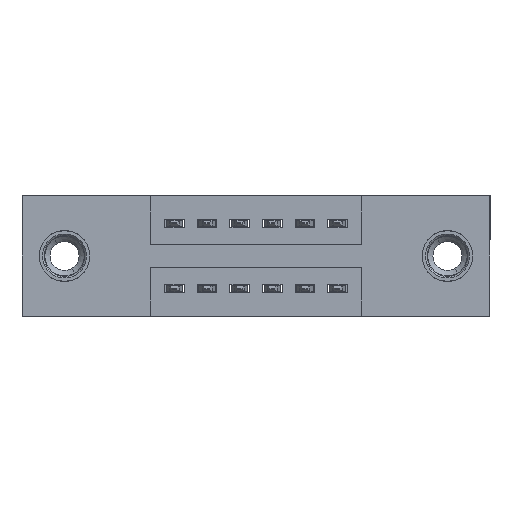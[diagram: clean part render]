
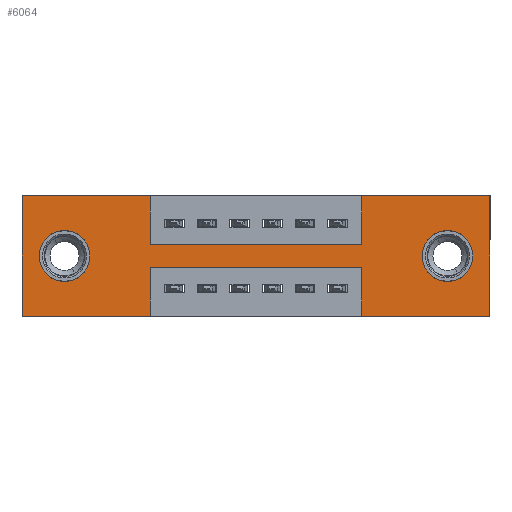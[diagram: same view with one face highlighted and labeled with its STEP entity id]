
A CAD part, front view. The second image highlights one B-rep face of the part: STEP entity #6064.
In plain terms, the highlighted planar face has unit normal (0, -1, 0).
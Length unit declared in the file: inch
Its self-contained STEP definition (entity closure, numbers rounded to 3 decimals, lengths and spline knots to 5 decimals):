
#124 = DIRECTION ( 'NONE',  ( 1., 0., 0. ) ) ;
#131 = LINE ( 'NONE', #4079, #9655 ) ;
#132 = EDGE_CURVE ( 'NONE', #5124, #314, #8219, .T. ) ;
#210 = ORIENTED_EDGE ( 'NONE', *, *, #3829, .T. ) ;
#260 = VECTOR ( 'NONE', #7945, 39.37008 ) ;
#314 = VERTEX_POINT ( 'NONE', #3733 ) ;
#321 = VERTEX_POINT ( 'NONE', #10904 ) ;
#384 = VERTEX_POINT ( 'NONE', #8227 ) ;
#517 = CARTESIAN_POINT ( 'NONE',  ( 1.0425, 0., -0.37 ) ) ;
#525 = EDGE_LOOP ( 'NONE', ( #11361, #210 ) ) ;
#572 = ORIENTED_EDGE ( 'NONE', *, *, #3975, .F. ) ;
#603 = CARTESIAN_POINT ( 'NONE',  ( 1.305, 0., -0.263 ) ) ;
#633 = AXIS2_PLACEMENT_3D ( 'NONE', #4261, #10539, #5156 ) ;
#740 = CIRCLE ( 'NONE', #633, 0.078 ) ;
#840 = CARTESIAN_POINT ( 'NONE',  ( 1.435, 0., 0. ) ) ;
#897 = DIRECTION ( 'NONE',  ( 0., -1., 0. ) ) ;
#974 = CARTESIAN_POINT ( 'NONE',  ( 0., 0., -0.37 ) ) ;
#1023 = ORIENTED_EDGE ( 'NONE', *, *, #4430, .T. ) ;
#1068 = DIRECTION ( 'NONE',  ( 0., 0., -1. ) ) ;
#1197 = LINE ( 'NONE', #10492, #3129 ) ;
#1275 = DIRECTION ( 'NONE',  ( 0., 1., 0. ) ) ;
#1791 = CARTESIAN_POINT ( 'NONE',  ( 0.3925, 0., 0. ) ) ;
#1823 = ORIENTED_EDGE ( 'NONE', *, *, #5217, .F. ) ;
#1884 = VERTEX_POINT ( 'NONE', #4316 ) ;
#1911 = VECTOR ( 'NONE', #6548, 39.37008 ) ;
#2116 = EDGE_CURVE ( 'NONE', #11554, #9631, #9535, .T. ) ;
#2135 = EDGE_CURVE ( 'NONE', #5106, #6953, #5011, .T. ) ;
#2216 = LINE ( 'NONE', #974, #1911 ) ;
#2228 = DIRECTION ( 'NONE',  ( 0., 1., 0. ) ) ;
#2556 = LINE ( 'NONE', #517, #260 ) ;
#2621 = VECTOR ( 'NONE', #3770, 39.37008 ) ;
#2711 = VECTOR ( 'NONE', #6985, 39.37008 ) ;
#2813 = ORIENTED_EDGE ( 'NONE', *, *, #6141, .F. ) ;
#2816 = EDGE_CURVE ( 'NONE', #314, #321, #131, .T. ) ;
#2923 = DIRECTION ( 'NONE',  ( 0., 0., -1. ) ) ;
#3078 = VECTOR ( 'NONE', #5081, 39.37008 ) ;
#3116 = CIRCLE ( 'NONE', #3929, 0.078 ) ;
#3129 = VECTOR ( 'NONE', #4170, 39.37008 ) ;
#3727 = CARTESIAN_POINT ( 'NONE',  ( 0., 0., -0.37 ) ) ;
#3733 = CARTESIAN_POINT ( 'NONE',  ( 0.3925, 0., -0.22 ) ) ;
#3770 = DIRECTION ( 'NONE',  ( 1., 0., 0. ) ) ;
#3829 = EDGE_CURVE ( 'NONE', #9293, #8934, #11154, .T. ) ;
#3920 = EDGE_CURVE ( 'NONE', #8699, #5106, #1197, .T. ) ;
#3929 = AXIS2_PLACEMENT_3D ( 'NONE', #6838, #1275, #7749 ) ;
#3975 = EDGE_CURVE ( 'NONE', #9783, #5124, #2556, .T. ) ;
#3978 = CARTESIAN_POINT ( 'NONE',  ( 0., 0., 0. ) ) ;
#4079 = CARTESIAN_POINT ( 'NONE',  ( 0.3925, 0., -0.37 ) ) ;
#4170 = DIRECTION ( 'NONE',  ( 1., 0., 0. ) ) ;
#4261 = CARTESIAN_POINT ( 'NONE',  ( 0.13, 0., -0.185 ) ) ;
#4316 = CARTESIAN_POINT ( 'NONE',  ( 1.0425, 0., -0.15 ) ) ;
#4330 = DIRECTION ( 'NONE',  ( -1., 0., 0. ) ) ;
#4430 = EDGE_CURVE ( 'NONE', #10887, #6436, #3116, .T. ) ;
#4585 = CARTESIAN_POINT ( 'NONE',  ( 1.0425, 0., -0.37 ) ) ;
#4748 = VECTOR ( 'NONE', #1068, 39.37008 ) ;
#4793 = ORIENTED_EDGE ( 'NONE', *, *, #2135, .F. ) ;
#4940 = FACE_BOUND ( 'NONE', #10703, .T. ) ;
#5011 = LINE ( 'NONE', #840, #4748 ) ;
#5038 = LINE ( 'NONE', #6460, #2621 ) ;
#5081 = DIRECTION ( 'NONE',  ( -1., 0., 0. ) ) ;
#5106 = VERTEX_POINT ( 'NONE', #10468 ) ;
#5108 = VECTOR ( 'NONE', #9379, 39.37008 ) ;
#5124 = VERTEX_POINT ( 'NONE', #10499 ) ;
#5156 = DIRECTION ( 'NONE',  ( 0., 0., 1. ) ) ;
#5217 = EDGE_CURVE ( 'NONE', #6953, #9783, #8957, .T. ) ;
#5424 = ORIENTED_EDGE ( 'NONE', *, *, #10143, .T. ) ;
#5445 = CARTESIAN_POINT ( 'NONE',  ( 1.305, 0., -0.185 ) ) ;
#5556 = EDGE_CURVE ( 'NONE', #384, #11554, #10025, .T. ) ;
#5749 = CARTESIAN_POINT ( 'NONE',  ( 0., 0., 0. ) ) ;
#6064 = ADVANCED_FACE ( 'NONE', ( #11798, #4940, #7673 ), #6459, .T. ) ;
#6141 = EDGE_CURVE ( 'NONE', #321, #10696, #2216, .T. ) ;
#6148 = CARTESIAN_POINT ( 'NONE',  ( 0., 0., -0.37 ) ) ;
#6224 = ORIENTED_EDGE ( 'NONE', *, *, #132, .F. ) ;
#6347 = DIRECTION ( 'NONE',  ( 0., 0., -1. ) ) ;
#6409 = ORIENTED_EDGE ( 'NONE', *, *, #3920, .F. ) ;
#6436 = VERTEX_POINT ( 'NONE', #7156 ) ;
#6459 = PLANE ( 'NONE',  #8289 ) ;
#6460 = CARTESIAN_POINT ( 'NONE',  ( 0.3925, 0., -0.15 ) ) ;
#6548 = DIRECTION ( 'NONE',  ( -1., 0., 0. ) ) ;
#6838 = CARTESIAN_POINT ( 'NONE',  ( 0.13, 0., -0.185 ) ) ;
#6940 = CARTESIAN_POINT ( 'NONE',  ( 1.0425, 0., 0. ) ) ;
#6953 = VERTEX_POINT ( 'NONE', #7176 ) ;
#6985 = DIRECTION ( 'NONE',  ( 0., 0., 1. ) ) ;
#7033 = EDGE_CURVE ( 'NONE', #8934, #9293, #7363, .T. ) ;
#7156 = CARTESIAN_POINT ( 'NONE',  ( 0.13, 0., -0.107 ) ) ;
#7157 = EDGE_LOOP ( 'NONE', ( #7839, #6224, #572, #1823, #4793, #6409, #11469, #9533, #9194, #7658, #8920, #2813 ) ) ;
#7176 = CARTESIAN_POINT ( 'NONE',  ( 1.435, 0., -0.37 ) ) ;
#7181 = VECTOR ( 'NONE', #8354, 39.37008 ) ;
#7363 = CIRCLE ( 'NONE', #8212, 0.078 ) ;
#7392 = DIRECTION ( 'NONE',  ( 0., 0., -1. ) ) ;
#7561 = LINE ( 'NONE', #3978, #5108 ) ;
#7574 = LINE ( 'NONE', #7886, #2711 ) ;
#7658 = ORIENTED_EDGE ( 'NONE', *, *, #5556, .F. ) ;
#7673 = FACE_OUTER_BOUND ( 'NONE', #7157, .T. ) ;
#7725 = CARTESIAN_POINT ( 'NONE',  ( 1.305, 0., -0.185 ) ) ;
#7729 = EDGE_CURVE ( 'NONE', #9631, #1884, #5038, .T. ) ;
#7749 = DIRECTION ( 'NONE',  ( 0., 0., 1. ) ) ;
#7839 = ORIENTED_EDGE ( 'NONE', *, *, #2816, .F. ) ;
#7886 = CARTESIAN_POINT ( 'NONE',  ( 1.0425, 0., 0. ) ) ;
#7945 = DIRECTION ( 'NONE',  ( 0., 0., 1. ) ) ;
#7959 = VECTOR ( 'NONE', #124, 39.37008 ) ;
#8048 = CARTESIAN_POINT ( 'NONE',  ( 0.3925, 0., -0.15 ) ) ;
#8212 = AXIS2_PLACEMENT_3D ( 'NONE', #5445, #11685, #6347 ) ;
#8219 = LINE ( 'NONE', #10598, #3078 ) ;
#8227 = CARTESIAN_POINT ( 'NONE',  ( 0., 0., 0. ) ) ;
#8289 = AXIS2_PLACEMENT_3D ( 'NONE', #3727, #897, #7392 ) ;
#8327 = CARTESIAN_POINT ( 'NONE',  ( 0.3925, 0., 0. ) ) ;
#8354 = DIRECTION ( 'NONE',  ( 0., 0., -1. ) ) ;
#8627 = CARTESIAN_POINT ( 'NONE',  ( 0., 0., -0.37 ) ) ;
#8632 = DIRECTION ( 'NONE',  ( 0., 0., -1. ) ) ;
#8699 = VERTEX_POINT ( 'NONE', #6940 ) ;
#8920 = ORIENTED_EDGE ( 'NONE', *, *, #10611, .F. ) ;
#8934 = VERTEX_POINT ( 'NONE', #11845 ) ;
#8957 = LINE ( 'NONE', #6148, #11542 ) ;
#9194 = ORIENTED_EDGE ( 'NONE', *, *, #2116, .F. ) ;
#9293 = VERTEX_POINT ( 'NONE', #603 ) ;
#9379 = DIRECTION ( 'NONE',  ( 0., 0., 1. ) ) ;
#9533 = ORIENTED_EDGE ( 'NONE', *, *, #7729, .F. ) ;
#9535 = LINE ( 'NONE', #8327, #7181 ) ;
#9631 = VERTEX_POINT ( 'NONE', #8048 ) ;
#9655 = VECTOR ( 'NONE', #2923, 39.37008 ) ;
#9783 = VERTEX_POINT ( 'NONE', #4585 ) ;
#10024 = AXIS2_PLACEMENT_3D ( 'NONE', #7725, #2228, #8632 ) ;
#10025 = LINE ( 'NONE', #5749, #7959 ) ;
#10143 = EDGE_CURVE ( 'NONE', #6436, #10887, #740, .T. ) ;
#10152 = EDGE_CURVE ( 'NONE', #1884, #8699, #7574, .T. ) ;
#10468 = CARTESIAN_POINT ( 'NONE',  ( 1.435, 0., 0. ) ) ;
#10492 = CARTESIAN_POINT ( 'NONE',  ( 0., 0., 0. ) ) ;
#10499 = CARTESIAN_POINT ( 'NONE',  ( 1.0425, 0., -0.22 ) ) ;
#10539 = DIRECTION ( 'NONE',  ( 0., 1., 0. ) ) ;
#10598 = CARTESIAN_POINT ( 'NONE',  ( 0.3925, 0., -0.22 ) ) ;
#10611 = EDGE_CURVE ( 'NONE', #10696, #384, #7561, .T. ) ;
#10696 = VERTEX_POINT ( 'NONE', #8627 ) ;
#10703 = EDGE_LOOP ( 'NONE', ( #5424, #1023 ) ) ;
#10796 = CARTESIAN_POINT ( 'NONE',  ( 0.13, 0., -0.263 ) ) ;
#10887 = VERTEX_POINT ( 'NONE', #10796 ) ;
#10904 = CARTESIAN_POINT ( 'NONE',  ( 0.3925, 0., -0.37 ) ) ;
#11154 = CIRCLE ( 'NONE', #10024, 0.078 ) ;
#11361 = ORIENTED_EDGE ( 'NONE', *, *, #7033, .T. ) ;
#11469 = ORIENTED_EDGE ( 'NONE', *, *, #10152, .F. ) ;
#11542 = VECTOR ( 'NONE', #4330, 39.37008 ) ;
#11554 = VERTEX_POINT ( 'NONE', #1791 ) ;
#11685 = DIRECTION ( 'NONE',  ( 0., 1., 0. ) ) ;
#11798 = FACE_BOUND ( 'NONE', #525, .T. ) ;
#11845 = CARTESIAN_POINT ( 'NONE',  ( 1.305, 0., -0.107 ) ) ;
